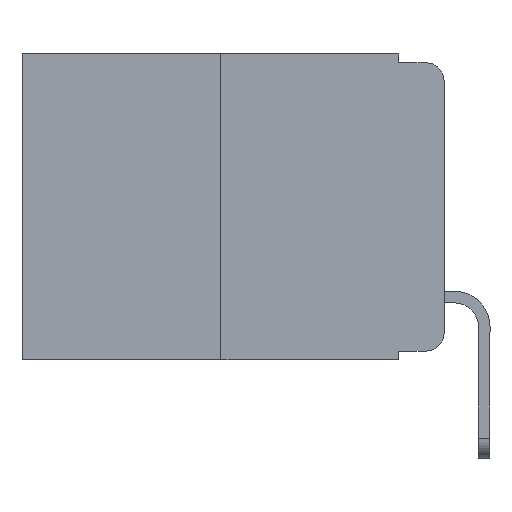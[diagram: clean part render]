
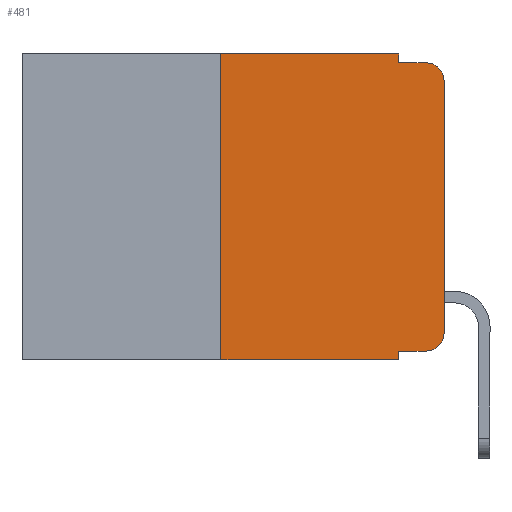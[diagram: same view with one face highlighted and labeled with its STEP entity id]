
A CAD part, left-side view. The second image highlights one B-rep face of the part: STEP entity #481.
In plain terms, the highlighted planar face has unit normal (-1, 0, 0).
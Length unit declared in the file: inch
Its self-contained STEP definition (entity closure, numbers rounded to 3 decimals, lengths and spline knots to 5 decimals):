
#481 = ADVANCED_FACE ( 'NONE', ( #16190 ), #16861, .F. ) ;
#980 = CARTESIAN_POINT ( 'NONE',  ( 0., 0.051, -0.01 ) ) ;
#2235 = VECTOR ( 'NONE', #13398, 39.37008 ) ;
#2565 = EDGE_CURVE ( 'NONE', #3259, #14119, #10892, .T. ) ;
#2600 = VECTOR ( 'NONE', #16504, 39.37008 ) ;
#3259 = VERTEX_POINT ( 'NONE', #18402 ) ;
#3447 = ORIENTED_EDGE ( 'NONE', *, *, #2565, .F. ) ;
#3538 = CARTESIAN_POINT ( 'NONE',  ( 0., 0.473, 0. ) ) ;
#4108 = CARTESIAN_POINT ( 'NONE',  ( 0., 0.051, 0. ) ) ;
#4194 = AXIS2_PLACEMENT_3D ( 'NONE', #16509, #15571, #15707 ) ;
#4659 = CARTESIAN_POINT ( 'NONE',  ( 0., 0.051, -0.01 ) ) ;
#5402 = DIRECTION ( 'NONE',  ( 0., 0., 1. ) ) ;
#5736 = CARTESIAN_POINT ( 'NONE',  ( 0., 0.473, -0.343 ) ) ;
#5818 = VERTEX_POINT ( 'NONE', #10051 ) ;
#6373 = DIRECTION ( 'NONE',  ( 0., -1., 0. ) ) ;
#6469 = ORIENTED_EDGE ( 'NONE', *, *, #8748, .T. ) ;
#6576 = CARTESIAN_POINT ( 'NONE',  ( 0., 0.02, -0.313 ) ) ;
#7166 = VERTEX_POINT ( 'NONE', #11555 ) ;
#7415 = LINE ( 'NONE', #9054, #11581 ) ;
#7505 = DIRECTION ( 'NONE',  ( 0., -1., 0. ) ) ;
#7869 = DIRECTION ( 'NONE',  ( -1., 0., 0. ) ) ;
#7880 = CARTESIAN_POINT ( 'NONE',  ( 0., 0.25, -0.343 ) ) ;
#8157 = DIRECTION ( 'NONE',  ( 0., 0., -1. ) ) ;
#8314 = VERTEX_POINT ( 'NONE', #980 ) ;
#8459 = ORIENTED_EDGE ( 'NONE', *, *, #13217, .F. ) ;
#8748 = EDGE_CURVE ( 'NONE', #7166, #9977, #17040, .T. ) ;
#8888 = LINE ( 'NONE', #14854, #12460 ) ;
#9054 = CARTESIAN_POINT ( 'NONE',  ( 0., 0.25, 0. ) ) ;
#9453 = ORIENTED_EDGE ( 'NONE', *, *, #14490, .T. ) ;
#9567 = EDGE_CURVE ( 'NONE', #14353, #5818, #14663, .T. ) ;
#9958 = LINE ( 'NONE', #4659, #17013 ) ;
#9977 = VERTEX_POINT ( 'NONE', #14420 ) ;
#10051 = CARTESIAN_POINT ( 'NONE',  ( 0., 0.051, -0.343 ) ) ;
#10450 = VECTOR ( 'NONE', #14712, 39.37008 ) ;
#10605 = DIRECTION ( 'NONE',  ( 0., 0., 1. ) ) ;
#10692 = EDGE_CURVE ( 'NONE', #11955, #19106, #8888, .T. ) ;
#10799 = DIRECTION ( 'NONE',  ( 0., 0., -1. ) ) ;
#10892 = LINE ( 'NONE', #3538, #2600 ) ;
#11555 = CARTESIAN_POINT ( 'NONE',  ( 0., 0., -0.03 ) ) ;
#11581 = VECTOR ( 'NONE', #10605, 39.37008 ) ;
#11955 = VERTEX_POINT ( 'NONE', #19641 ) ;
#12067 = ORIENTED_EDGE ( 'NONE', *, *, #16395, .F. ) ;
#12460 = VECTOR ( 'NONE', #7505, 39.37008 ) ;
#12974 = CIRCLE ( 'NONE', #16365, 0.02 ) ;
#12990 = CARTESIAN_POINT ( 'NONE',  ( 0., 0., -0.313 ) ) ;
#13217 = EDGE_CURVE ( 'NONE', #11955, #5818, #19380, .T. ) ;
#13398 = DIRECTION ( 'NONE',  ( 0., 0., -1. ) ) ;
#14119 = VERTEX_POINT ( 'NONE', #4108 ) ;
#14353 = VERTEX_POINT ( 'NONE', #7880 ) ;
#14386 = EDGE_CURVE ( 'NONE', #8314, #9977, #9958, .T. ) ;
#14420 = CARTESIAN_POINT ( 'NONE',  ( 0., 0.02, -0.01 ) ) ;
#14481 = CARTESIAN_POINT ( 'NONE',  ( 0., 0., 0. ) ) ;
#14490 = EDGE_CURVE ( 'NONE', #19106, #16854, #12974, .T. ) ;
#14663 = LINE ( 'NONE', #5736, #10450 ) ;
#14712 = DIRECTION ( 'NONE',  ( 0., -1., 0. ) ) ;
#14854 = CARTESIAN_POINT ( 'NONE',  ( 0., 0.051, -0.333 ) ) ;
#15040 = VECTOR ( 'NONE', #5402, 39.37008 ) ;
#15344 = VECTOR ( 'NONE', #10799, 39.37008 ) ;
#15360 = EDGE_LOOP ( 'NONE', ( #17628, #6469, #18059, #18476, #3447, #12067, #19319, #8459, #19733, #9453 ) ) ;
#15474 = LINE ( 'NONE', #14481, #15040 ) ;
#15571 = DIRECTION ( 'NONE',  ( 1., 0., 0. ) ) ;
#15707 = DIRECTION ( 'NONE',  ( 0., 0., -1. ) ) ;
#16098 = EDGE_CURVE ( 'NONE', #16854, #7166, #15474, .T. ) ;
#16190 = FACE_OUTER_BOUND ( 'NONE', #15360, .T. ) ;
#16365 = AXIS2_PLACEMENT_3D ( 'NONE', #6576, #16802, #8157 ) ;
#16395 = EDGE_CURVE ( 'NONE', #14353, #3259, #7415, .T. ) ;
#16504 = DIRECTION ( 'NONE',  ( 0., -1., 0. ) ) ;
#16509 = CARTESIAN_POINT ( 'NONE',  ( 0., 0.473, 0. ) ) ;
#16567 = CARTESIAN_POINT ( 'NONE',  ( 0., 0.02, -0.333 ) ) ;
#16568 = CARTESIAN_POINT ( 'NONE',  ( 0., 0.02, -0.03 ) ) ;
#16802 = DIRECTION ( 'NONE',  ( -1., 0., 0. ) ) ;
#16854 = VERTEX_POINT ( 'NONE', #12990 ) ;
#16861 = PLANE ( 'NONE',  #4194 ) ;
#17013 = VECTOR ( 'NONE', #6373, 39.37008 ) ;
#17040 = CIRCLE ( 'NONE', #17143, 0.02 ) ;
#17116 = EDGE_CURVE ( 'NONE', #14119, #8314, #18010, .T. ) ;
#17143 = AXIS2_PLACEMENT_3D ( 'NONE', #16568, #7869, #17941 ) ;
#17628 = ORIENTED_EDGE ( 'NONE', *, *, #16098, .T. ) ;
#17785 = CARTESIAN_POINT ( 'NONE',  ( 0., 0.051, 0. ) ) ;
#17941 = DIRECTION ( 'NONE',  ( 0., 0., -1. ) ) ;
#18010 = LINE ( 'NONE', #18811, #2235 ) ;
#18059 = ORIENTED_EDGE ( 'NONE', *, *, #14386, .F. ) ;
#18402 = CARTESIAN_POINT ( 'NONE',  ( 0., 0.25, 0. ) ) ;
#18476 = ORIENTED_EDGE ( 'NONE', *, *, #17116, .F. ) ;
#18811 = CARTESIAN_POINT ( 'NONE',  ( 0., 0.051, 0. ) ) ;
#19106 = VERTEX_POINT ( 'NONE', #16567 ) ;
#19319 = ORIENTED_EDGE ( 'NONE', *, *, #9567, .T. ) ;
#19380 = LINE ( 'NONE', #17785, #15344 ) ;
#19641 = CARTESIAN_POINT ( 'NONE',  ( 0., 0.051, -0.333 ) ) ;
#19733 = ORIENTED_EDGE ( 'NONE', *, *, #10692, .T. ) ;
